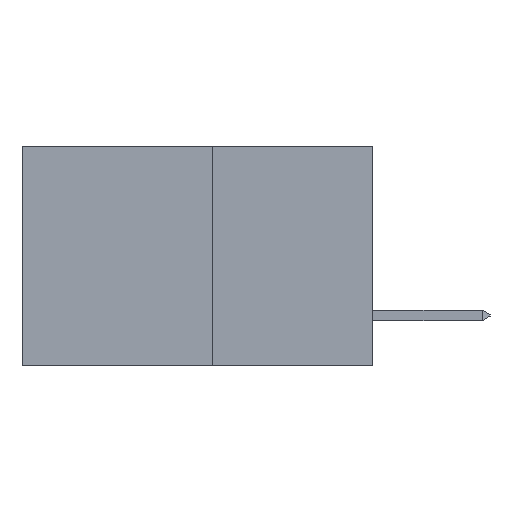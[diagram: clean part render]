
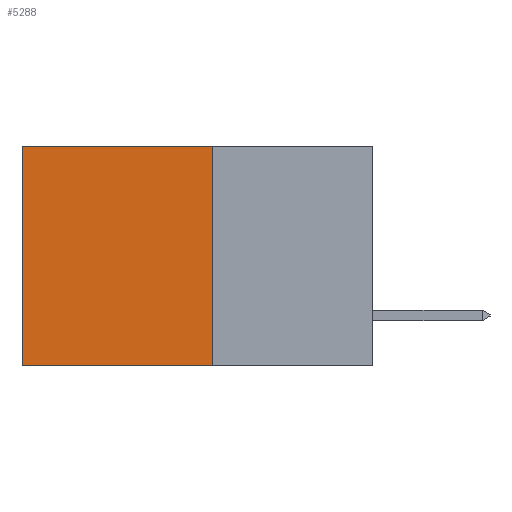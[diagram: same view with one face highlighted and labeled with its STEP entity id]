
A CAD part, left-side view. The second image highlights one B-rep face of the part: STEP entity #5288.
In plain terms, the highlighted planar face has unit normal (-1, 0, 0).
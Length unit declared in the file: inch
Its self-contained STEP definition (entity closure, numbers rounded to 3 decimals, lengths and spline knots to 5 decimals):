
#653 = DIRECTION ( 'NONE',  ( 0., 1., 0. ) ) ;
#1004 = EDGE_LOOP ( 'NONE', ( #9409, #13971, #5097, #3544 ) ) ;
#1961 = VECTOR ( 'NONE', #11956, 39.37008 ) ;
#1962 = DIRECTION ( 'NONE',  ( 0., 0., -1. ) ) ;
#2090 = DIRECTION ( 'NONE',  ( 1., 0., 0. ) ) ;
#2216 = CARTESIAN_POINT ( 'NONE',  ( 0.277, 0.27, -0.37 ) ) ;
#2270 = PLANE ( 'NONE',  #8523 ) ;
#2614 = LINE ( 'NONE', #5330, #10045 ) ;
#3224 = VERTEX_POINT ( 'NONE', #7377 ) ;
#3544 = ORIENTED_EDGE ( 'NONE', *, *, #7133, .T. ) ;
#4199 = LINE ( 'NONE', #4725, #14836 ) ;
#4725 = CARTESIAN_POINT ( 'NONE',  ( 0.277, 0.27, -0.37 ) ) ;
#5060 = CARTESIAN_POINT ( 'NONE',  ( 0.277, 0.59, -0.37 ) ) ;
#5097 = ORIENTED_EDGE ( 'NONE', *, *, #15950, .F. ) ;
#5185 = CARTESIAN_POINT ( 'NONE',  ( 0.277, 0.59, -0.37 ) ) ;
#5288 = ADVANCED_FACE ( 'NONE', ( #12116 ), #2270, .F. ) ;
#5330 = CARTESIAN_POINT ( 'NONE',  ( 0.277, 0.27, -0.37 ) ) ;
#6128 = DIRECTION ( 'NONE',  ( 0., 0., -1. ) ) ;
#6148 = VERTEX_POINT ( 'NONE', #5185 ) ;
#6212 = LINE ( 'NONE', #17932, #9437 ) ;
#7133 = EDGE_CURVE ( 'NONE', #12028, #3224, #6212, .T. ) ;
#7377 = CARTESIAN_POINT ( 'NONE',  ( 0.277, 0.59, 0. ) ) ;
#7471 = CARTESIAN_POINT ( 'NONE',  ( 0.277, 0.27, 0. ) ) ;
#8523 = AXIS2_PLACEMENT_3D ( 'NONE', #2216, #2090, #1962 ) ;
#9409 = ORIENTED_EDGE ( 'NONE', *, *, #16892, .T. ) ;
#9437 = VECTOR ( 'NONE', #653, 39.37008 ) ;
#10045 = VECTOR ( 'NONE', #14995, 39.37008 ) ;
#10947 = CARTESIAN_POINT ( 'NONE',  ( 0.277, 0.27, -0.37 ) ) ;
#11956 = DIRECTION ( 'NONE',  ( 0., 0., -1. ) ) ;
#12028 = VERTEX_POINT ( 'NONE', #7471 ) ;
#12116 = FACE_OUTER_BOUND ( 'NONE', #1004, .T. ) ;
#12994 = VERTEX_POINT ( 'NONE', #10947 ) ;
#13071 = LINE ( 'NONE', #5060, #1961 ) ;
#13971 = ORIENTED_EDGE ( 'NONE', *, *, #16246, .F. ) ;
#14836 = VECTOR ( 'NONE', #6128, 39.37008 ) ;
#14995 = DIRECTION ( 'NONE',  ( 0., 1., 0. ) ) ;
#15950 = EDGE_CURVE ( 'NONE', #12028, #12994, #4199, .T. ) ;
#16246 = EDGE_CURVE ( 'NONE', #12994, #6148, #2614, .T. ) ;
#16892 = EDGE_CURVE ( 'NONE', #3224, #6148, #13071, .T. ) ;
#17932 = CARTESIAN_POINT ( 'NONE',  ( 0.277, 0.27, 0. ) ) ;
